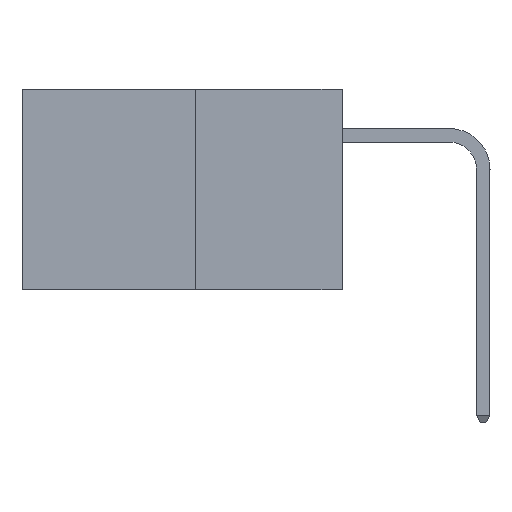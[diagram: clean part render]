
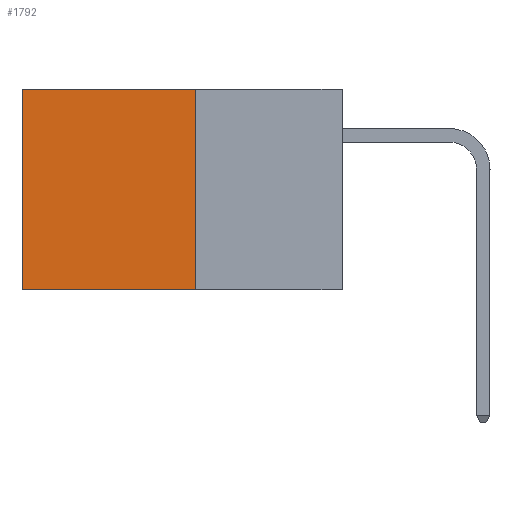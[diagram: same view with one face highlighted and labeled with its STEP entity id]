
A CAD part, left-side view. The second image highlights one B-rep face of the part: STEP entity #1792.
In plain terms, the highlighted planar face has unit normal (-1, 0, 0).
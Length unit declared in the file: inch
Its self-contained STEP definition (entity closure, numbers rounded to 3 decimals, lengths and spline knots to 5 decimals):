
#91 = DIRECTION ( 'NONE',  ( 0., 0., -1. ) ) ;
#529 = DIRECTION ( 'NONE',  ( 0., 0., -1. ) ) ;
#774 = CARTESIAN_POINT ( 'NONE',  ( 0.277, 0.27, 0. ) ) ;
#896 = ORIENTED_EDGE ( 'NONE', *, *, #1884, .T. ) ;
#910 = ORIENTED_EDGE ( 'NONE', *, *, #1195, .F. ) ;
#920 = ORIENTED_EDGE ( 'NONE', *, *, #5330, .F. ) ;
#938 = ORIENTED_EDGE ( 'NONE', *, *, #2657, .T. ) ;
#1195 = EDGE_CURVE ( 'NONE', #8749, #7281, #1257, .T. ) ;
#1257 = LINE ( 'NONE', #6178, #3462 ) ;
#1291 = VERTEX_POINT ( 'NONE', #774 ) ;
#1686 = DIRECTION ( 'NONE',  ( 0., 1., 0. ) ) ;
#1733 = LINE ( 'NONE', #8786, #5567 ) ;
#1765 = LINE ( 'NONE', #5874, #8369 ) ;
#1792 = ADVANCED_FACE ( 'NONE', ( #5267 ), #8580, .F. ) ;
#1884 = EDGE_CURVE ( 'NONE', #5702, #7281, #1765, .T. ) ;
#2096 = EDGE_LOOP ( 'NONE', ( #896, #910, #920, #938 ) ) ;
#2657 = EDGE_CURVE ( 'NONE', #1291, #5702, #1733, .T. ) ;
#3167 = CARTESIAN_POINT ( 'NONE',  ( 0.277, 0.27, -0.37 ) ) ;
#3462 = VECTOR ( 'NONE', #1686, 39.37008 ) ;
#3617 = DIRECTION ( 'NONE',  ( 0., 1., 0. ) ) ;
#4897 = VECTOR ( 'NONE', #91, 39.37008 ) ;
#4948 = DIRECTION ( 'NONE',  ( 0., 0., -1. ) ) ;
#5183 = CARTESIAN_POINT ( 'NONE',  ( 0.277, 0.59, -0.37 ) ) ;
#5192 = CARTESIAN_POINT ( 'NONE',  ( 0.277, 0.27, -0.37 ) ) ;
#5267 = FACE_OUTER_BOUND ( 'NONE', #2096, .T. ) ;
#5330 = EDGE_CURVE ( 'NONE', #1291, #8749, #6693, .T. ) ;
#5567 = VECTOR ( 'NONE', #3617, 39.37008 ) ;
#5702 = VERTEX_POINT ( 'NONE', #8631 ) ;
#5874 = CARTESIAN_POINT ( 'NONE',  ( 0.277, 0.59, -0.37 ) ) ;
#6178 = CARTESIAN_POINT ( 'NONE',  ( 0.277, 0.27, -0.37 ) ) ;
#6530 = CARTESIAN_POINT ( 'NONE',  ( 0.277, 0.27, -0.37 ) ) ;
#6693 = LINE ( 'NONE', #5192, #4897 ) ;
#6722 = AXIS2_PLACEMENT_3D ( 'NONE', #3167, #8699, #529 ) ;
#7281 = VERTEX_POINT ( 'NONE', #5183 ) ;
#8369 = VECTOR ( 'NONE', #4948, 39.37008 ) ;
#8580 = PLANE ( 'NONE',  #6722 ) ;
#8631 = CARTESIAN_POINT ( 'NONE',  ( 0.277, 0.59, 0. ) ) ;
#8699 = DIRECTION ( 'NONE',  ( 1., 0., 0. ) ) ;
#8749 = VERTEX_POINT ( 'NONE', #6530 ) ;
#8786 = CARTESIAN_POINT ( 'NONE',  ( 0.277, 0.27, 0. ) ) ;
